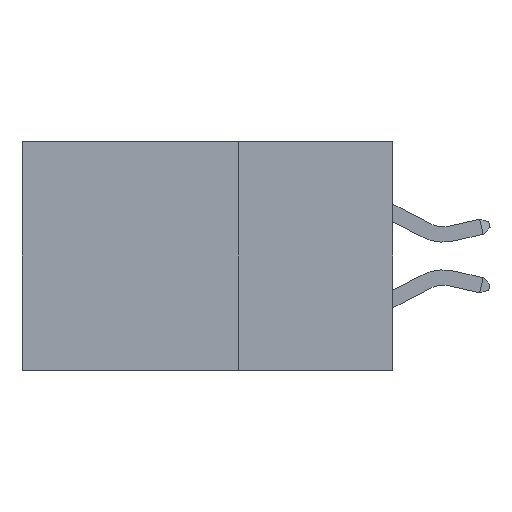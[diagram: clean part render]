
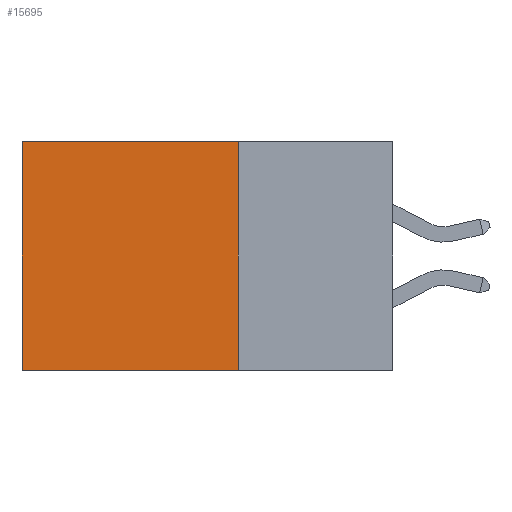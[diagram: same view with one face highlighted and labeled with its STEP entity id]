
A CAD part, left-side view. The second image highlights one B-rep face of the part: STEP entity #15695.
In plain terms, the highlighted planar face has unit normal (-1, 0, 0).
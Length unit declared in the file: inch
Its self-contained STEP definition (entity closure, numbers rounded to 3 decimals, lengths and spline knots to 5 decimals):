
#218 = ORIENTED_EDGE ( 'NONE', *, *, #27218, .T. ) ;
#639 = VECTOR ( 'NONE', #6969, 39.37008 ) ;
#2903 = LINE ( 'NONE', #10264, #3275 ) ;
#3275 = VECTOR ( 'NONE', #7858, 39.37008 ) ;
#3418 = DIRECTION ( 'NONE',  ( 1., 0., 0. ) ) ;
#6969 = DIRECTION ( 'NONE',  ( 0., 1., 0. ) ) ;
#7150 = ORIENTED_EDGE ( 'NONE', *, *, #23795, .F. ) ;
#7858 = DIRECTION ( 'NONE',  ( 0., 0., -1. ) ) ;
#7962 = CARTESIAN_POINT ( 'NONE',  ( 0.2875, 0.25, -0.37 ) ) ;
#8195 = ORIENTED_EDGE ( 'NONE', *, *, #11749, .F. ) ;
#8365 = FACE_OUTER_BOUND ( 'NONE', #23606, .T. ) ;
#10264 = CARTESIAN_POINT ( 'NONE',  ( 0.2875, 0.6, 0. ) ) ;
#11014 = CARTESIAN_POINT ( 'NONE',  ( 0.2875, 0.25, -0.37 ) ) ;
#11672 = VERTEX_POINT ( 'NONE', #16937 ) ;
#11749 = EDGE_CURVE ( 'NONE', #22050, #18288, #16238, .T. ) ;
#11761 = LINE ( 'NONE', #14014, #639 ) ;
#12326 = CARTESIAN_POINT ( 'NONE',  ( 0.2875, 0.25, 0. ) ) ;
#12445 = ORIENTED_EDGE ( 'NONE', *, *, #16023, .T. ) ;
#13429 = VECTOR ( 'NONE', #23419, 39.37008 ) ;
#14014 = CARTESIAN_POINT ( 'NONE',  ( 0.2875, 0.25, 0. ) ) ;
#14662 = DIRECTION ( 'NONE',  ( 0., 0., -1. ) ) ;
#15688 = CARTESIAN_POINT ( 'NONE',  ( 0.2875, 0.25, 0. ) ) ;
#15695 = ADVANCED_FACE ( 'NONE', ( #8365 ), #21445, .F. ) ;
#16023 = EDGE_CURVE ( 'NONE', #22050, #11672, #11761, .T. ) ;
#16238 = LINE ( 'NONE', #25567, #13429 ) ;
#16937 = CARTESIAN_POINT ( 'NONE',  ( 0.2875, 0.6, 0. ) ) ;
#18288 = VERTEX_POINT ( 'NONE', #7962 ) ;
#21445 = PLANE ( 'NONE',  #28154 ) ;
#21880 = LINE ( 'NONE', #11014, #26009 ) ;
#22050 = VERTEX_POINT ( 'NONE', #15688 ) ;
#23419 = DIRECTION ( 'NONE',  ( 0., 0., -1. ) ) ;
#23606 = EDGE_LOOP ( 'NONE', ( #218, #7150, #8195, #12445 ) ) ;
#23795 = EDGE_CURVE ( 'NONE', #18288, #28581, #21880, .T. ) ;
#25567 = CARTESIAN_POINT ( 'NONE',  ( 0.2875, 0.25, 0. ) ) ;
#26009 = VECTOR ( 'NONE', #26607, 39.37008 ) ;
#26150 = CARTESIAN_POINT ( 'NONE',  ( 0.2875, 0.6, -0.37 ) ) ;
#26607 = DIRECTION ( 'NONE',  ( 0., 1., 0. ) ) ;
#27218 = EDGE_CURVE ( 'NONE', #11672, #28581, #2903, .T. ) ;
#28154 = AXIS2_PLACEMENT_3D ( 'NONE', #12326, #3418, #14662 ) ;
#28581 = VERTEX_POINT ( 'NONE', #26150 ) ;
